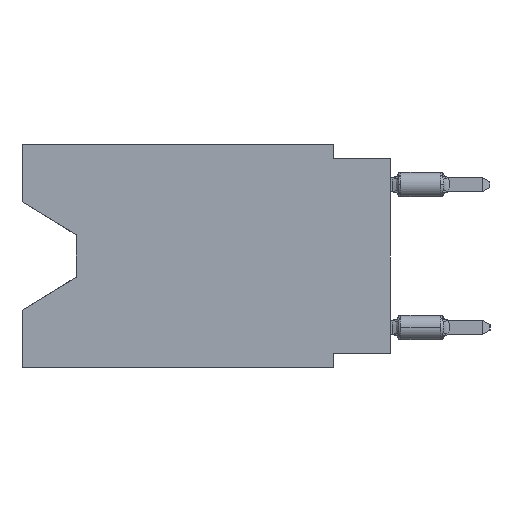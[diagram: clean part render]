
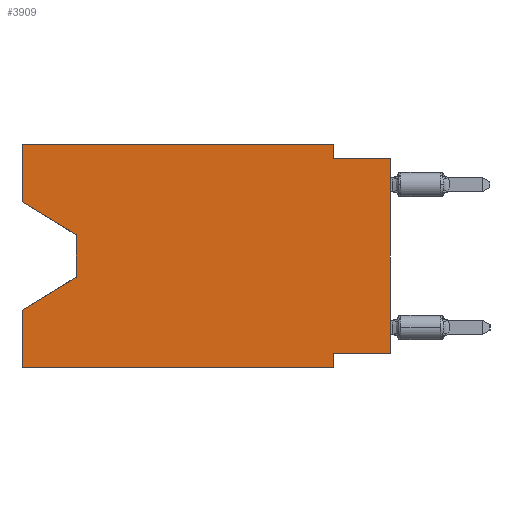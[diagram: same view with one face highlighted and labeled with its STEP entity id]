
A CAD part, left-side view. The second image highlights one B-rep face of the part: STEP entity #3909.
In plain terms, the highlighted planar face has unit normal (-1, 0, 0).
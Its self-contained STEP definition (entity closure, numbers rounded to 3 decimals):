
#51 = EDGE_CURVE ( 'NONE', #3205, #28782, #26231, .T. ) ;
#382 = CARTESIAN_POINT ( 'NONE',  ( 0., 16.383, 0. ) ) ;
#495 = VERTEX_POINT ( 'NONE', #31646 ) ;
#541 = EDGE_CURVE ( 'NONE', #13993, #19270, #21330, .T. ) ;
#1660 = CARTESIAN_POINT ( 'NONE',  ( 0., 13.97, -4.013 ) ) ;
#1816 = PLANE ( 'NONE',  #18300 ) ;
#1842 = DIRECTION ( 'NONE',  ( 0., -0.855, -0.519 ) ) ;
#2750 = CARTESIAN_POINT ( 'NONE',  ( 0., 16.383, -9.906 ) ) ;
#3205 = VERTEX_POINT ( 'NONE', #4671 ) ;
#3679 = VECTOR ( 'NONE', #16379, 1000. ) ;
#3909 = ADVANCED_FACE ( 'NONE', ( #7314 ), #1816, .F. ) ;
#4087 = VECTOR ( 'NONE', #32841, 1000. ) ;
#4671 = CARTESIAN_POINT ( 'NONE',  ( 0., 16.383, 0. ) ) ;
#4938 = LINE ( 'NONE', #28488, #24186 ) ;
#5350 = VERTEX_POINT ( 'NONE', #19904 ) ;
#5370 = LINE ( 'NONE', #382, #15559 ) ;
#5608 = CARTESIAN_POINT ( 'NONE',  ( 0., 2.54, 0. ) ) ;
#5707 = EDGE_CURVE ( 'NONE', #24139, #19732, #33474, .T. ) ;
#5737 = EDGE_CURVE ( 'NONE', #27459, #19270, #9574, .T. ) ;
#5867 = EDGE_CURVE ( 'NONE', #13660, #8103, #4938, .T. ) ;
#6065 = VECTOR ( 'NONE', #14365, 1000. ) ;
#6136 = VECTOR ( 'NONE', #13741, 1000. ) ;
#6227 = LINE ( 'NONE', #32529, #3679 ) ;
#6995 = LINE ( 'NONE', #33487, #21707 ) ;
#7314 = FACE_OUTER_BOUND ( 'NONE', #15514, .T. ) ;
#7730 = EDGE_CURVE ( 'NONE', #13993, #5350, #6227, .T. ) ;
#8005 = DIRECTION ( 'NONE',  ( 0., -1., 0. ) ) ;
#8103 = VERTEX_POINT ( 'NONE', #20832 ) ;
#8277 = LINE ( 'NONE', #18756, #24614 ) ;
#9222 = LINE ( 'NONE', #14371, #18431 ) ;
#9574 = LINE ( 'NONE', #30368, #20920 ) ;
#10207 = CARTESIAN_POINT ( 'NONE',  ( 0., 13.97, -4.013 ) ) ;
#11033 = EDGE_CURVE ( 'NONE', #32161, #8103, #6995, .T. ) ;
#11071 = CARTESIAN_POINT ( 'NONE',  ( 0., 2.54, -0.635 ) ) ;
#11703 = ORIENTED_EDGE ( 'NONE', *, *, #12449, .T. ) ;
#12449 = EDGE_CURVE ( 'NONE', #495, #24139, #9222, .T. ) ;
#12849 = DIRECTION ( 'NONE',  ( 0., -1., 0. ) ) ;
#13438 = DIRECTION ( 'NONE',  ( 0., 0.855, -0.519 ) ) ;
#13660 = VERTEX_POINT ( 'NONE', #29746 ) ;
#13741 = DIRECTION ( 'NONE',  ( 0., -1., 0. ) ) ;
#13993 = VERTEX_POINT ( 'NONE', #2750 ) ;
#14365 = DIRECTION ( 'NONE',  ( 0., 0., -1. ) ) ;
#14371 = CARTESIAN_POINT ( 'NONE',  ( 0., 16.383, -2.546 ) ) ;
#14749 = CARTESIAN_POINT ( 'NONE',  ( 0., 2.54, -9.906 ) ) ;
#14877 = EDGE_CURVE ( 'NONE', #495, #3205, #5370, .T. ) ;
#14892 = VECTOR ( 'NONE', #8005, 1000. ) ;
#15221 = CARTESIAN_POINT ( 'NONE',  ( 0., 16.383, 0. ) ) ;
#15514 = EDGE_LOOP ( 'NONE', ( #11703, #31191, #27544, #20960, #30783, #25844, #30892, #25106, #18083, #20933, #27043, #26195 ) ) ;
#15559 = VECTOR ( 'NONE', #26349, 1000. ) ;
#15813 = EDGE_CURVE ( 'NONE', #13660, #27459, #25696, .T. ) ;
#16005 = EDGE_CURVE ( 'NONE', #28782, #32161, #27839, .T. ) ;
#16379 = DIRECTION ( 'NONE',  ( 0., 0., 1. ) ) ;
#18083 = ORIENTED_EDGE ( 'NONE', *, *, #11033, .F. ) ;
#18300 = AXIS2_PLACEMENT_3D ( 'NONE', #15221, #20211, #30178 ) ;
#18431 = VECTOR ( 'NONE', #1842, 1000. ) ;
#18756 = CARTESIAN_POINT ( 'NONE',  ( 0., 13.97, -5.893 ) ) ;
#19270 = VERTEX_POINT ( 'NONE', #14749 ) ;
#19732 = VERTEX_POINT ( 'NONE', #30457 ) ;
#19883 = EDGE_CURVE ( 'NONE', #19732, #5350, #8277, .T. ) ;
#19904 = CARTESIAN_POINT ( 'NONE',  ( 0., 16.383, -7.36 ) ) ;
#19935 = CARTESIAN_POINT ( 'NONE',  ( 0., 2.54, 0. ) ) ;
#20211 = DIRECTION ( 'NONE',  ( 1., 0., 0. ) ) ;
#20537 = CARTESIAN_POINT ( 'NONE',  ( 0., 0., -9.271 ) ) ;
#20588 = DIRECTION ( 'NONE',  ( 0., 0., 1. ) ) ;
#20832 = CARTESIAN_POINT ( 'NONE',  ( 0., 0., -0.635 ) ) ;
#20920 = VECTOR ( 'NONE', #25382, 1000. ) ;
#20933 = ORIENTED_EDGE ( 'NONE', *, *, #16005, .F. ) ;
#20960 = ORIENTED_EDGE ( 'NONE', *, *, #7730, .F. ) ;
#21330 = LINE ( 'NONE', #33582, #6136 ) ;
#21707 = VECTOR ( 'NONE', #12849, 1000. ) ;
#24139 = VERTEX_POINT ( 'NONE', #10207 ) ;
#24186 = VECTOR ( 'NONE', #20588, 1000. ) ;
#24614 = VECTOR ( 'NONE', #13438, 1000. ) ;
#25106 = ORIENTED_EDGE ( 'NONE', *, *, #5867, .T. ) ;
#25382 = DIRECTION ( 'NONE',  ( 0., 0., -1. ) ) ;
#25696 = LINE ( 'NONE', #20537, #33762 ) ;
#25844 = ORIENTED_EDGE ( 'NONE', *, *, #5737, .F. ) ;
#26065 = CARTESIAN_POINT ( 'NONE',  ( 0., 16.383, 0. ) ) ;
#26195 = ORIENTED_EDGE ( 'NONE', *, *, #14877, .F. ) ;
#26231 = LINE ( 'NONE', #26065, #14892 ) ;
#26349 = DIRECTION ( 'NONE',  ( 0., 0., 1. ) ) ;
#26747 = CARTESIAN_POINT ( 'NONE',  ( 0., 2.54, -9.271 ) ) ;
#27043 = ORIENTED_EDGE ( 'NONE', *, *, #51, .F. ) ;
#27459 = VERTEX_POINT ( 'NONE', #26747 ) ;
#27544 = ORIENTED_EDGE ( 'NONE', *, *, #19883, .T. ) ;
#27839 = LINE ( 'NONE', #19935, #4087 ) ;
#28488 = CARTESIAN_POINT ( 'NONE',  ( 0., 0., 0. ) ) ;
#28782 = VERTEX_POINT ( 'NONE', #5608 ) ;
#29746 = CARTESIAN_POINT ( 'NONE',  ( 0., 0., -9.271 ) ) ;
#30178 = DIRECTION ( 'NONE',  ( 0., 0., -1. ) ) ;
#30368 = CARTESIAN_POINT ( 'NONE',  ( 0., 2.54, -9.906 ) ) ;
#30457 = CARTESIAN_POINT ( 'NONE',  ( 0., 13.97, -5.893 ) ) ;
#30506 = DIRECTION ( 'NONE',  ( 0., 1., 0. ) ) ;
#30783 = ORIENTED_EDGE ( 'NONE', *, *, #541, .T. ) ;
#30892 = ORIENTED_EDGE ( 'NONE', *, *, #15813, .F. ) ;
#31191 = ORIENTED_EDGE ( 'NONE', *, *, #5707, .T. ) ;
#31646 = CARTESIAN_POINT ( 'NONE',  ( 0., 16.383, -2.546 ) ) ;
#32161 = VERTEX_POINT ( 'NONE', #11071 ) ;
#32529 = CARTESIAN_POINT ( 'NONE',  ( 0., 16.383, 0. ) ) ;
#32841 = DIRECTION ( 'NONE',  ( 0., 0., -1. ) ) ;
#33474 = LINE ( 'NONE', #1660, #6065 ) ;
#33487 = CARTESIAN_POINT ( 'NONE',  ( 0., 0., -0.635 ) ) ;
#33582 = CARTESIAN_POINT ( 'NONE',  ( 0., 16.383, -9.906 ) ) ;
#33762 = VECTOR ( 'NONE', #30506, 1000. ) ;
